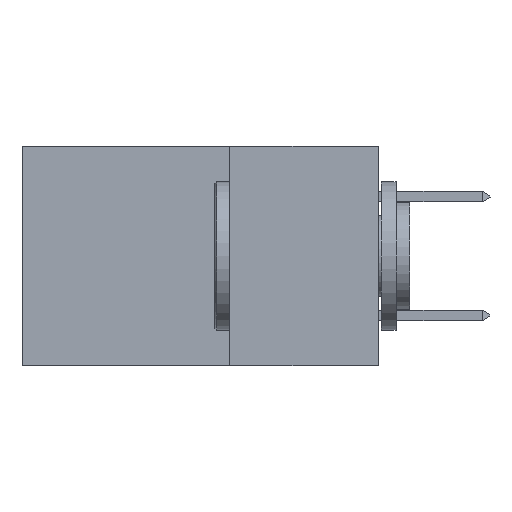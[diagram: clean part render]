
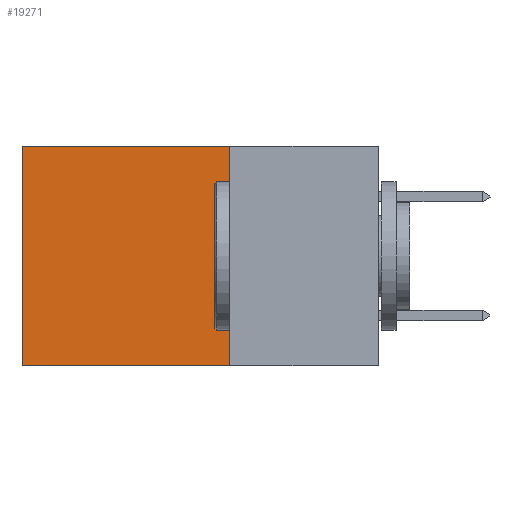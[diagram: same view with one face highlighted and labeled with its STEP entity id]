
A CAD part, left-side view. The second image highlights one B-rep face of the part: STEP entity #19271.
In plain terms, the highlighted planar face has unit normal (-1, 0, 0).
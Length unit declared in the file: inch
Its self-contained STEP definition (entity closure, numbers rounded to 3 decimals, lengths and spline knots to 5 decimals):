
#46 = VERTEX_POINT ( 'NONE', #19768 ) ;
#1513 = CARTESIAN_POINT ( 'NONE',  ( 0.298, 0.25, 0. ) ) ;
#2052 = EDGE_LOOP ( 'NONE', ( #5604, #7062, #14451, #13528 ) ) ;
#3658 = DIRECTION ( 'NONE',  ( 0., 0., -1. ) ) ;
#3873 = VECTOR ( 'NONE', #3658, 39.37008 ) ;
#4135 = DIRECTION ( 'NONE',  ( 1., 0., 0. ) ) ;
#5604 = ORIENTED_EDGE ( 'NONE', *, *, #10812, .T. ) ;
#6526 = FACE_OUTER_BOUND ( 'NONE', #2052, .T. ) ;
#6918 = VERTEX_POINT ( 'NONE', #19453 ) ;
#7062 = ORIENTED_EDGE ( 'NONE', *, *, #8623, .F. ) ;
#7387 = LINE ( 'NONE', #15091, #18209 ) ;
#7820 = PLANE ( 'NONE',  #11158 ) ;
#7864 = DIRECTION ( 'NONE',  ( 0., 1., 0. ) ) ;
#7880 = VERTEX_POINT ( 'NONE', #1513 ) ;
#8055 = DIRECTION ( 'NONE',  ( 0., 1., 0. ) ) ;
#8480 = LINE ( 'NONE', #9670, #10931 ) ;
#8623 = EDGE_CURVE ( 'NONE', #6918, #46, #7387, .T. ) ;
#9003 = LINE ( 'NONE', #14088, #3873 ) ;
#9338 = CARTESIAN_POINT ( 'NONE',  ( 0.298, 0.25, 0. ) ) ;
#9670 = CARTESIAN_POINT ( 'NONE',  ( 0.298, 0.6, 0. ) ) ;
#10198 = VECTOR ( 'NONE', #7864, 39.37008 ) ;
#10248 = VERTEX_POINT ( 'NONE', #13788 ) ;
#10812 = EDGE_CURVE ( 'NONE', #10248, #46, #8480, .T. ) ;
#10931 = VECTOR ( 'NONE', #16618, 39.37008 ) ;
#11158 = AXIS2_PLACEMENT_3D ( 'NONE', #9338, #4135, #12738 ) ;
#12738 = DIRECTION ( 'NONE',  ( 0., 0., -1. ) ) ;
#13528 = ORIENTED_EDGE ( 'NONE', *, *, #16749, .T. ) ;
#13788 = CARTESIAN_POINT ( 'NONE',  ( 0.298, 0.6, 0. ) ) ;
#14088 = CARTESIAN_POINT ( 'NONE',  ( 0.298, 0.25, 0. ) ) ;
#14451 = ORIENTED_EDGE ( 'NONE', *, *, #21990, .F. ) ;
#15091 = CARTESIAN_POINT ( 'NONE',  ( 0.298, 0.25, -0.37 ) ) ;
#16618 = DIRECTION ( 'NONE',  ( 0., 0., -1. ) ) ;
#16648 = CARTESIAN_POINT ( 'NONE',  ( 0.298, 0.25, 0. ) ) ;
#16749 = EDGE_CURVE ( 'NONE', #7880, #10248, #21795, .T. ) ;
#18209 = VECTOR ( 'NONE', #8055, 39.37008 ) ;
#19271 = ADVANCED_FACE ( 'NONE', ( #6526 ), #7820, .F. ) ;
#19453 = CARTESIAN_POINT ( 'NONE',  ( 0.298, 0.25, -0.37 ) ) ;
#19768 = CARTESIAN_POINT ( 'NONE',  ( 0.298, 0.6, -0.37 ) ) ;
#21795 = LINE ( 'NONE', #16648, #10198 ) ;
#21990 = EDGE_CURVE ( 'NONE', #7880, #6918, #9003, .T. ) ;
